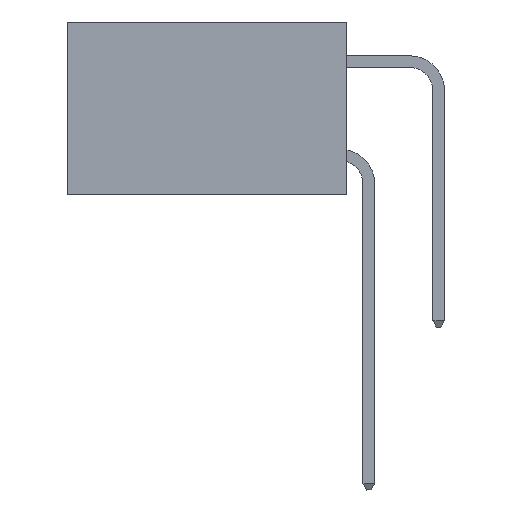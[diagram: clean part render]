
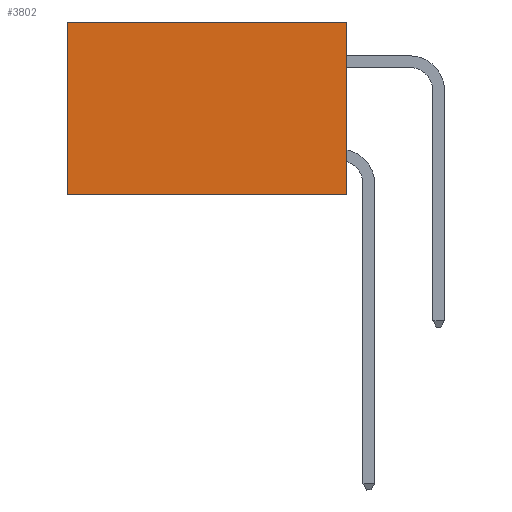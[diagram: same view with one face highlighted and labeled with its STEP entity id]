
A CAD part, left-side view. The second image highlights one B-rep face of the part: STEP entity #3802.
In plain terms, the highlighted planar face has unit normal (-1, 0, 0).
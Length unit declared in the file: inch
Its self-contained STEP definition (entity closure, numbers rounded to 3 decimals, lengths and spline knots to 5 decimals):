
#1899 = VERTEX_POINT ( 'NONE', #2029 ) ;
#2029 = CARTESIAN_POINT ( 'NONE',  ( 0.2875, 0.6, 0. ) ) ;
#3501 = VECTOR ( 'NONE', #22760, 39.37008 ) ;
#3802 = ADVANCED_FACE ( 'NONE', ( #27625 ), #8985, .F. ) ;
#6229 = VECTOR ( 'NONE', #15053, 39.37008 ) ;
#7996 = LINE ( 'NONE', #37424, #34807 ) ;
#8610 = ORIENTED_EDGE ( 'NONE', *, *, #26571, .F. ) ;
#8985 = PLANE ( 'NONE',  #22870 ) ;
#9499 = ORIENTED_EDGE ( 'NONE', *, *, #14188, .T. ) ;
#9822 = EDGE_CURVE ( 'NONE', #18792, #1899, #22126, .T. ) ;
#11431 = CARTESIAN_POINT ( 'NONE',  ( 0.2875, 0., -0.37 ) ) ;
#11555 = ORIENTED_EDGE ( 'NONE', *, *, #9822, .T. ) ;
#12478 = DIRECTION ( 'NONE',  ( 0., 0., -1. ) ) ;
#12902 = DIRECTION ( 'NONE',  ( 0., 1., 0. ) ) ;
#14188 = EDGE_CURVE ( 'NONE', #1899, #22782, #24417, .T. ) ;
#15053 = DIRECTION ( 'NONE',  ( 0., 0., -1. ) ) ;
#15522 = LINE ( 'NONE', #18394, #6229 ) ;
#17016 = EDGE_CURVE ( 'NONE', #35636, #22782, #7996, .T. ) ;
#18394 = CARTESIAN_POINT ( 'NONE',  ( 0.2875, 0., 0. ) ) ;
#18792 = VERTEX_POINT ( 'NONE', #36781 ) ;
#19338 = CARTESIAN_POINT ( 'NONE',  ( 0.2875, 0., 0. ) ) ;
#21824 = EDGE_LOOP ( 'NONE', ( #9499, #29646, #8610, #11555 ) ) ;
#22126 = LINE ( 'NONE', #40202, #3501 ) ;
#22760 = DIRECTION ( 'NONE',  ( 0., 1., 0. ) ) ;
#22782 = VERTEX_POINT ( 'NONE', #43467 ) ;
#22870 = AXIS2_PLACEMENT_3D ( 'NONE', #19338, #33461, #12478 ) ;
#24417 = LINE ( 'NONE', #39753, #33911 ) ;
#26571 = EDGE_CURVE ( 'NONE', #18792, #35636, #15522, .T. ) ;
#27625 = FACE_OUTER_BOUND ( 'NONE', #21824, .T. ) ;
#29646 = ORIENTED_EDGE ( 'NONE', *, *, #17016, .F. ) ;
#32865 = DIRECTION ( 'NONE',  ( 0., 0., -1. ) ) ;
#33461 = DIRECTION ( 'NONE',  ( 1., 0., 0. ) ) ;
#33911 = VECTOR ( 'NONE', #32865, 39.37008 ) ;
#34807 = VECTOR ( 'NONE', #12902, 39.37008 ) ;
#35636 = VERTEX_POINT ( 'NONE', #11431 ) ;
#36781 = CARTESIAN_POINT ( 'NONE',  ( 0.2875, 0., 0. ) ) ;
#37424 = CARTESIAN_POINT ( 'NONE',  ( 0.2875, 0., -0.37 ) ) ;
#39753 = CARTESIAN_POINT ( 'NONE',  ( 0.2875, 0.6, 0. ) ) ;
#40202 = CARTESIAN_POINT ( 'NONE',  ( 0.2875, 0., 0. ) ) ;
#43467 = CARTESIAN_POINT ( 'NONE',  ( 0.2875, 0.6, -0.37 ) ) ;
